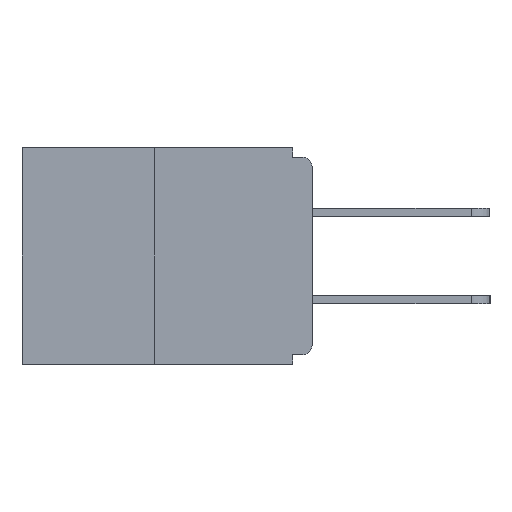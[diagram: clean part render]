
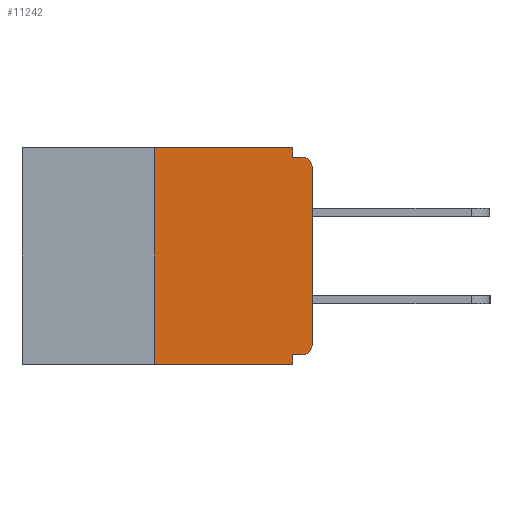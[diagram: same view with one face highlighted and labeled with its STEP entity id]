
A CAD part, left-side view. The second image highlights one B-rep face of the part: STEP entity #11242.
In plain terms, the highlighted planar face has unit normal (-1, 0, 0).
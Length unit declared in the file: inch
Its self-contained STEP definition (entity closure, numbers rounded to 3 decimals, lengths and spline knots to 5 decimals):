
#60 = CIRCLE ( 'NONE', #5099, 0.015 ) ;
#270 = CARTESIAN_POINT ( 'NONE',  ( 0., 0.46, 0. ) ) ;
#276 = CARTESIAN_POINT ( 'NONE',  ( 0., 0.031, 0. ) ) ;
#309 = CARTESIAN_POINT ( 'NONE',  ( 0., 0.015, -0.015 ) ) ;
#392 = ORIENTED_EDGE ( 'NONE', *, *, #9470, .F. ) ;
#405 = ORIENTED_EDGE ( 'NONE', *, *, #3405, .F. ) ;
#406 = VERTEX_POINT ( 'NONE', #309 ) ;
#451 = ORIENTED_EDGE ( 'NONE', *, *, #13347, .F. ) ;
#728 = EDGE_CURVE ( 'NONE', #5053, #10741, #12396, .T. ) ;
#732 = CARTESIAN_POINT ( 'NONE',  ( 0., 0., -0.313 ) ) ;
#839 = EDGE_CURVE ( 'NONE', #5053, #4293, #60, .T. ) ;
#927 = CARTESIAN_POINT ( 'NONE',  ( 0., 0.031, -0.328 ) ) ;
#1323 = DIRECTION ( 'NONE',  ( 0., 0., 1. ) ) ;
#1623 = ORIENTED_EDGE ( 'NONE', *, *, #9039, .T. ) ;
#1913 = EDGE_CURVE ( 'NONE', #8645, #13313, #8774, .T. ) ;
#2048 = VERTEX_POINT ( 'NONE', #5760 ) ;
#2160 = DIRECTION ( 'NONE',  ( 0., 1., 0. ) ) ;
#2405 = LINE ( 'NONE', #2742, #3582 ) ;
#2736 = ORIENTED_EDGE ( 'NONE', *, *, #7763, .T. ) ;
#2742 = CARTESIAN_POINT ( 'NONE',  ( 0., 0.031, -0.343 ) ) ;
#3177 = ORIENTED_EDGE ( 'NONE', *, *, #839, .T. ) ;
#3256 = LINE ( 'NONE', #4929, #11312 ) ;
#3405 = EDGE_CURVE ( 'NONE', #12713, #8645, #5124, .T. ) ;
#3537 = CARTESIAN_POINT ( 'NONE',  ( 0., 0., -0.015 ) ) ;
#3557 = FACE_OUTER_BOUND ( 'NONE', #5435, .T. ) ;
#3582 = VECTOR ( 'NONE', #13646, 39.37008 ) ;
#4223 = VECTOR ( 'NONE', #1323, 39.37008 ) ;
#4293 = VERTEX_POINT ( 'NONE', #732 ) ;
#4335 = DIRECTION ( 'NONE',  ( -1., 0., 0. ) ) ;
#4548 = LINE ( 'NONE', #10272, #4223 ) ;
#4612 = DIRECTION ( 'NONE',  ( 0., 0., -1. ) ) ;
#4891 = EDGE_CURVE ( 'NONE', #4293, #5081, #4548, .T. ) ;
#4929 = CARTESIAN_POINT ( 'NONE',  ( 0., 0.46, -0.343 ) ) ;
#5053 = VERTEX_POINT ( 'NONE', #11789 ) ;
#5058 = DIRECTION ( 'NONE',  ( 0., 0., -1. ) ) ;
#5081 = VERTEX_POINT ( 'NONE', #7447 ) ;
#5099 = AXIS2_PLACEMENT_3D ( 'NONE', #8712, #10201, #4612 ) ;
#5124 = LINE ( 'NONE', #5962, #6497 ) ;
#5435 = EDGE_LOOP ( 'NONE', ( #11989, #405, #1623, #392, #9064, #3177, #7165, #2736, #451, #8350 ) ) ;
#5556 = CARTESIAN_POINT ( 'NONE',  ( 0., 0., -0.328 ) ) ;
#5619 = CARTESIAN_POINT ( 'NONE',  ( 0., 0.25, -0.343 ) ) ;
#5760 = CARTESIAN_POINT ( 'NONE',  ( 0., 0.031, -0.015 ) ) ;
#5962 = CARTESIAN_POINT ( 'NONE',  ( 0., 0.25, 0. ) ) ;
#6497 = VECTOR ( 'NONE', #9026, 39.37008 ) ;
#6642 = DIRECTION ( 'NONE',  ( 0., 0., -1. ) ) ;
#6829 = DIRECTION ( 'NONE',  ( 0., -1., 0. ) ) ;
#7165 = ORIENTED_EDGE ( 'NONE', *, *, #4891, .T. ) ;
#7447 = CARTESIAN_POINT ( 'NONE',  ( 0., 0., -0.03 ) ) ;
#7664 = VERTEX_POINT ( 'NONE', #12976 ) ;
#7677 = CARTESIAN_POINT ( 'NONE',  ( 0., 0.015, -0.03 ) ) ;
#7763 = EDGE_CURVE ( 'NONE', #5081, #406, #13801, .T. ) ;
#8018 = DIRECTION ( 'NONE',  ( 0., 0., -1. ) ) ;
#8350 = ORIENTED_EDGE ( 'NONE', *, *, #13332, .F. ) ;
#8631 = VECTOR ( 'NONE', #6829, 39.37008 ) ;
#8645 = VERTEX_POINT ( 'NONE', #9512 ) ;
#8712 = CARTESIAN_POINT ( 'NONE',  ( 0., 0.015, -0.313 ) ) ;
#8774 = LINE ( 'NONE', #270, #9491 ) ;
#9026 = DIRECTION ( 'NONE',  ( 0., 0., 1. ) ) ;
#9039 = EDGE_CURVE ( 'NONE', #12713, #7664, #3256, .T. ) ;
#9064 = ORIENTED_EDGE ( 'NONE', *, *, #728, .F. ) ;
#9470 = EDGE_CURVE ( 'NONE', #10741, #7664, #2405, .T. ) ;
#9491 = VECTOR ( 'NONE', #10039, 39.37008 ) ;
#9512 = CARTESIAN_POINT ( 'NONE',  ( 0., 0.25, 0. ) ) ;
#10039 = DIRECTION ( 'NONE',  ( 0., -1., 0. ) ) ;
#10201 = DIRECTION ( 'NONE',  ( -1., 0., 0. ) ) ;
#10272 = CARTESIAN_POINT ( 'NONE',  ( 0., 0., 0. ) ) ;
#10576 = AXIS2_PLACEMENT_3D ( 'NONE', #7677, #4335, #6642 ) ;
#10694 = LINE ( 'NONE', #276, #13983 ) ;
#10741 = VERTEX_POINT ( 'NONE', #927 ) ;
#11242 = ADVANCED_FACE ( 'NONE', ( #3557 ), #12674, .F. ) ;
#11312 = VECTOR ( 'NONE', #13719, 39.37008 ) ;
#11612 = CARTESIAN_POINT ( 'NONE',  ( 0., 0.46, 0. ) ) ;
#11709 = DIRECTION ( 'NONE',  ( 1., 0., 0. ) ) ;
#11789 = CARTESIAN_POINT ( 'NONE',  ( 0., 0.015, -0.328 ) ) ;
#11989 = ORIENTED_EDGE ( 'NONE', *, *, #1913, .F. ) ;
#12027 = CARTESIAN_POINT ( 'NONE',  ( 0., 0.031, 0. ) ) ;
#12396 = LINE ( 'NONE', #5556, #13072 ) ;
#12414 = LINE ( 'NONE', #3537, #8631 ) ;
#12674 = PLANE ( 'NONE',  #13167 ) ;
#12713 = VERTEX_POINT ( 'NONE', #5619 ) ;
#12976 = CARTESIAN_POINT ( 'NONE',  ( 0., 0.031, -0.343 ) ) ;
#13072 = VECTOR ( 'NONE', #2160, 39.37008 ) ;
#13167 = AXIS2_PLACEMENT_3D ( 'NONE', #11612, #11709, #5058 ) ;
#13313 = VERTEX_POINT ( 'NONE', #12027 ) ;
#13332 = EDGE_CURVE ( 'NONE', #13313, #2048, #10694, .T. ) ;
#13347 = EDGE_CURVE ( 'NONE', #2048, #406, #12414, .T. ) ;
#13646 = DIRECTION ( 'NONE',  ( 0., 0., -1. ) ) ;
#13719 = DIRECTION ( 'NONE',  ( 0., -1., 0. ) ) ;
#13801 = CIRCLE ( 'NONE', #10576, 0.015 ) ;
#13983 = VECTOR ( 'NONE', #8018, 39.37008 ) ;
